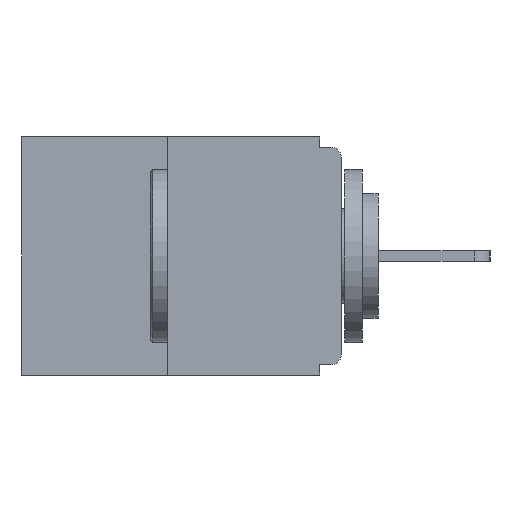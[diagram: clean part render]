
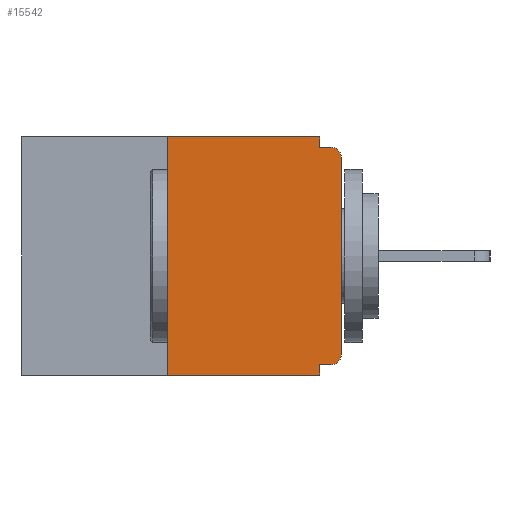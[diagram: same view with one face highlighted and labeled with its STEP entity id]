
A CAD part, left-side view. The second image highlights one B-rep face of the part: STEP entity #15542.
In plain terms, the highlighted planar face has unit normal (-1, 0, 0).
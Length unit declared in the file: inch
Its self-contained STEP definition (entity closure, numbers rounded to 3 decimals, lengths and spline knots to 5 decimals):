
#125 = LINE ( 'NONE', #11030, #9283 ) ;
#312 = LINE ( 'NONE', #11423, #6048 ) ;
#386 = DIRECTION ( 'NONE',  ( -1., 0., 0. ) ) ;
#393 = CIRCLE ( 'NONE', #18267, 0.015 ) ;
#620 = CARTESIAN_POINT ( 'NONE',  ( 0., 0.031, -0.015 ) ) ;
#1008 = VERTEX_POINT ( 'NONE', #6052 ) ;
#1010 = ORIENTED_EDGE ( 'NONE', *, *, #10352, .F. ) ;
#1065 = VERTEX_POINT ( 'NONE', #3503 ) ;
#1113 = DIRECTION ( 'NONE',  ( 0., -1., 0. ) ) ;
#1258 = EDGE_CURVE ( 'NONE', #16140, #1065, #11943, .T. ) ;
#1380 = PLANE ( 'NONE',  #2377 ) ;
#1738 = DIRECTION ( 'NONE',  ( 0., 0., -1. ) ) ;
#2227 = LINE ( 'NONE', #9653, #19241 ) ;
#2377 = AXIS2_PLACEMENT_3D ( 'NONE', #6243, #17137, #16841 ) ;
#2509 = VERTEX_POINT ( 'NONE', #4200 ) ;
#2587 = CARTESIAN_POINT ( 'NONE',  ( 0., 0., 0. ) ) ;
#2750 = ORIENTED_EDGE ( 'NONE', *, *, #12392, .T. ) ;
#3168 = ORIENTED_EDGE ( 'NONE', *, *, #14890, .F. ) ;
#3503 = CARTESIAN_POINT ( 'NONE',  ( 0., 0., -0.03 ) ) ;
#4089 = CARTESIAN_POINT ( 'NONE',  ( 0., 0.015, -0.328 ) ) ;
#4200 = CARTESIAN_POINT ( 'NONE',  ( 0., 0.031, 0. ) ) ;
#4229 = ORIENTED_EDGE ( 'NONE', *, *, #18768, .F. ) ;
#4237 = ORIENTED_EDGE ( 'NONE', *, *, #8215, .T. ) ;
#4526 = VECTOR ( 'NONE', #1113, 39.37008 ) ;
#4581 = CARTESIAN_POINT ( 'NONE',  ( 0., 0.031, -0.328 ) ) ;
#5052 = VECTOR ( 'NONE', #15560, 39.37008 ) ;
#5890 = AXIS2_PLACEMENT_3D ( 'NONE', #7936, #386, #1738 ) ;
#5904 = VERTEX_POINT ( 'NONE', #16400 ) ;
#6048 = VECTOR ( 'NONE', #14278, 39.37008 ) ;
#6052 = CARTESIAN_POINT ( 'NONE',  ( 0., 0.25, -0.343 ) ) ;
#6218 = VECTOR ( 'NONE', #7395, 39.37008 ) ;
#6243 = CARTESIAN_POINT ( 'NONE',  ( 0., 0.46, 0. ) ) ;
#6308 = LINE ( 'NONE', #15578, #17861 ) ;
#6842 = VERTEX_POINT ( 'NONE', #12179 ) ;
#7395 = DIRECTION ( 'NONE',  ( 0., 0., -1. ) ) ;
#7936 = CARTESIAN_POINT ( 'NONE',  ( 0., 0.015, -0.313 ) ) ;
#8215 = EDGE_CURVE ( 'NONE', #1065, #13302, #393, .T. ) ;
#8580 = DIRECTION ( 'NONE',  ( 0., 0., 1. ) ) ;
#9258 = CARTESIAN_POINT ( 'NONE',  ( 0., 0.46, -0.343 ) ) ;
#9283 = VECTOR ( 'NONE', #19613, 39.37008 ) ;
#9503 = CARTESIAN_POINT ( 'NONE',  ( 0., 0.031, -0.343 ) ) ;
#9653 = CARTESIAN_POINT ( 'NONE',  ( 0., 0., -0.328 ) ) ;
#10076 = VERTEX_POINT ( 'NONE', #4089 ) ;
#10077 = VERTEX_POINT ( 'NONE', #620 ) ;
#10246 = EDGE_LOOP ( 'NONE', ( #16808, #16716, #10832, #12555, #3168, #2750, #10624, #4237, #1010, #4229 ) ) ;
#10352 = EDGE_CURVE ( 'NONE', #10077, #13302, #6308, .T. ) ;
#10380 = LINE ( 'NONE', #14963, #4526 ) ;
#10596 = EDGE_CURVE ( 'NONE', #6842, #2509, #10380, .T. ) ;
#10624 = ORIENTED_EDGE ( 'NONE', *, *, #1258, .T. ) ;
#10832 = ORIENTED_EDGE ( 'NONE', *, *, #18546, .T. ) ;
#10978 = LINE ( 'NONE', #9258, #5052 ) ;
#11030 = CARTESIAN_POINT ( 'NONE',  ( 0., 0.25, 0. ) ) ;
#11092 = VECTOR ( 'NONE', #8580, 39.37008 ) ;
#11100 = CIRCLE ( 'NONE', #5890, 0.015 ) ;
#11147 = DIRECTION ( 'NONE',  ( 0., 0., -1. ) ) ;
#11423 = CARTESIAN_POINT ( 'NONE',  ( 0., 0.031, 0. ) ) ;
#11943 = LINE ( 'NONE', #2587, #11092 ) ;
#12179 = CARTESIAN_POINT ( 'NONE',  ( 0., 0.25, 0. ) ) ;
#12392 = EDGE_CURVE ( 'NONE', #10076, #16140, #11100, .T. ) ;
#12555 = ORIENTED_EDGE ( 'NONE', *, *, #14368, .F. ) ;
#12560 = LINE ( 'NONE', #9503, #6218 ) ;
#13302 = VERTEX_POINT ( 'NONE', #17628 ) ;
#14278 = DIRECTION ( 'NONE',  ( 0., 0., -1. ) ) ;
#14368 = EDGE_CURVE ( 'NONE', #19080, #5904, #12560, .T. ) ;
#14663 = CARTESIAN_POINT ( 'NONE',  ( 0., 0., -0.313 ) ) ;
#14890 = EDGE_CURVE ( 'NONE', #10076, #19080, #2227, .T. ) ;
#14963 = CARTESIAN_POINT ( 'NONE',  ( 0., 0.46, 0. ) ) ;
#15110 = FACE_OUTER_BOUND ( 'NONE', #10246, .T. ) ;
#15542 = ADVANCED_FACE ( 'NONE', ( #15110 ), #1380, .F. ) ;
#15560 = DIRECTION ( 'NONE',  ( 0., -1., 0. ) ) ;
#15578 = CARTESIAN_POINT ( 'NONE',  ( 0., 0., -0.015 ) ) ;
#15861 = DIRECTION ( 'NONE',  ( 0., 1., 0. ) ) ;
#15982 = DIRECTION ( 'NONE',  ( 0., -1., 0. ) ) ;
#16140 = VERTEX_POINT ( 'NONE', #14663 ) ;
#16400 = CARTESIAN_POINT ( 'NONE',  ( 0., 0.031, -0.343 ) ) ;
#16716 = ORIENTED_EDGE ( 'NONE', *, *, #20052, .F. ) ;
#16808 = ORIENTED_EDGE ( 'NONE', *, *, #10596, .F. ) ;
#16841 = DIRECTION ( 'NONE',  ( 0., 0., -1. ) ) ;
#17137 = DIRECTION ( 'NONE',  ( 1., 0., 0. ) ) ;
#17454 = CARTESIAN_POINT ( 'NONE',  ( 0., 0.015, -0.03 ) ) ;
#17628 = CARTESIAN_POINT ( 'NONE',  ( 0., 0.015, -0.015 ) ) ;
#17861 = VECTOR ( 'NONE', #15982, 39.37008 ) ;
#18267 = AXIS2_PLACEMENT_3D ( 'NONE', #17454, #19079, #11147 ) ;
#18546 = EDGE_CURVE ( 'NONE', #1008, #5904, #10978, .T. ) ;
#18768 = EDGE_CURVE ( 'NONE', #2509, #10077, #312, .T. ) ;
#19079 = DIRECTION ( 'NONE',  ( -1., 0., 0. ) ) ;
#19080 = VERTEX_POINT ( 'NONE', #4581 ) ;
#19241 = VECTOR ( 'NONE', #15861, 39.37008 ) ;
#19613 = DIRECTION ( 'NONE',  ( 0., 0., 1. ) ) ;
#20052 = EDGE_CURVE ( 'NONE', #1008, #6842, #125, .T. ) ;
